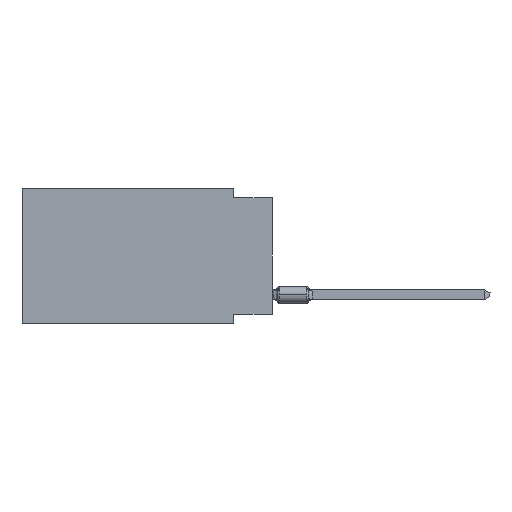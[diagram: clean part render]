
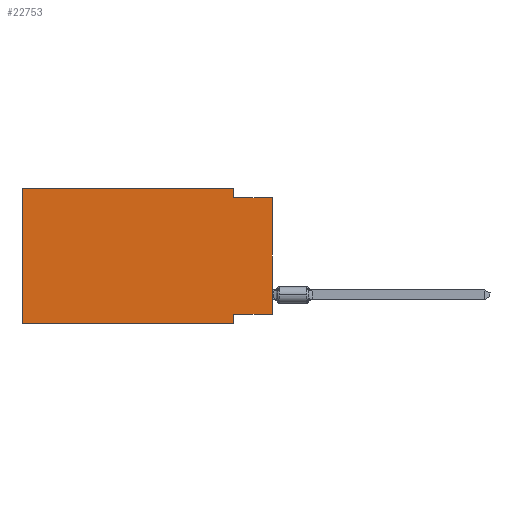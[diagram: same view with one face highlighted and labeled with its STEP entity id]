
A CAD part, left-side view. The second image highlights one B-rep face of the part: STEP entity #22753.
In plain terms, the highlighted planar face has unit normal (-1, 0, 0).
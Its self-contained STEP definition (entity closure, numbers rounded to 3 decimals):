
#332 = CARTESIAN_POINT ( 'NONE',  ( 0., 16.383, 0. ) ) ;
#1500 = ORIENTED_EDGE ( 'NONE', *, *, #2528, .T. ) ;
#1837 = VECTOR ( 'NONE', #15474, 1000. ) ;
#2460 = CARTESIAN_POINT ( 'NONE',  ( 0., 16.383, 0. ) ) ;
#2461 = VERTEX_POINT ( 'NONE', #23174 ) ;
#2528 = EDGE_CURVE ( 'NONE', #26982, #2461, #13024, .T. ) ;
#2749 = AXIS2_PLACEMENT_3D ( 'NONE', #332, #3429, #8899 ) ;
#3429 = DIRECTION ( 'NONE',  ( 1., 0., 0. ) ) ;
#3939 = DIRECTION ( 'NONE',  ( 0., -1., 0. ) ) ;
#4595 = DIRECTION ( 'NONE',  ( 0., 0., 1. ) ) ;
#4811 = VECTOR ( 'NONE', #4595, 1000. ) ;
#4900 = VERTEX_POINT ( 'NONE', #9694 ) ;
#5397 = CARTESIAN_POINT ( 'NONE',  ( 0., 0., -8.255 ) ) ;
#5995 = CARTESIAN_POINT ( 'NONE',  ( 0., 2.54, -8.89 ) ) ;
#6486 = EDGE_CURVE ( 'NONE', #4900, #34462, #22879, .T. ) ;
#7127 = ORIENTED_EDGE ( 'NONE', *, *, #11390, .F. ) ;
#7798 = VECTOR ( 'NONE', #11660, 1000. ) ;
#7998 = VECTOR ( 'NONE', #3939, 1000. ) ;
#8899 = DIRECTION ( 'NONE',  ( 0., 0., -1. ) ) ;
#9694 = CARTESIAN_POINT ( 'NONE',  ( 0., 2.54, -8.255 ) ) ;
#9794 = CARTESIAN_POINT ( 'NONE',  ( 0., 2.54, 0. ) ) ;
#10689 = VECTOR ( 'NONE', #33989, 1000. ) ;
#11288 = LINE ( 'NONE', #30801, #7798 ) ;
#11390 = EDGE_CURVE ( 'NONE', #14086, #2461, #34971, .T. ) ;
#11660 = DIRECTION ( 'NONE',  ( 0., 0., -1. ) ) ;
#11772 = LINE ( 'NONE', #5397, #16528 ) ;
#11944 = VERTEX_POINT ( 'NONE', #2460 ) ;
#12345 = EDGE_CURVE ( 'NONE', #11944, #24610, #33671, .T. ) ;
#12576 = EDGE_CURVE ( 'NONE', #30050, #34462, #32544, .T. ) ;
#13024 = LINE ( 'NONE', #13560, #20866 ) ;
#13560 = CARTESIAN_POINT ( 'NONE',  ( 0., 0., 0. ) ) ;
#14086 = VERTEX_POINT ( 'NONE', #18644 ) ;
#14142 = DIRECTION ( 'NONE',  ( 0., 1., 0. ) ) ;
#15474 = DIRECTION ( 'NONE',  ( 0., -1., 0. ) ) ;
#15601 = ORIENTED_EDGE ( 'NONE', *, *, #12345, .F. ) ;
#16215 = ORIENTED_EDGE ( 'NONE', *, *, #6486, .F. ) ;
#16327 = CARTESIAN_POINT ( 'NONE',  ( 0., 16.383, -8.89 ) ) ;
#16528 = VECTOR ( 'NONE', #14142, 1000. ) ;
#18141 = CARTESIAN_POINT ( 'NONE',  ( 0., 16.383, -8.89 ) ) ;
#18644 = CARTESIAN_POINT ( 'NONE',  ( 0., 2.54, -0.635 ) ) ;
#18817 = CARTESIAN_POINT ( 'NONE',  ( 0., 16.383, 0. ) ) ;
#18971 = EDGE_CURVE ( 'NONE', #26982, #4900, #11772, .T. ) ;
#19433 = ORIENTED_EDGE ( 'NONE', *, *, #27596, .F. ) ;
#19725 = ORIENTED_EDGE ( 'NONE', *, *, #12576, .T. ) ;
#20866 = VECTOR ( 'NONE', #30154, 1000. ) ;
#20907 = ORIENTED_EDGE ( 'NONE', *, *, #35634, .F. ) ;
#22368 = DIRECTION ( 'NONE',  ( 0., -1., 0. ) ) ;
#22753 = ADVANCED_FACE ( 'NONE', ( #34238 ), #31503, .F. ) ;
#22879 = LINE ( 'NONE', #28519, #10689 ) ;
#23174 = CARTESIAN_POINT ( 'NONE',  ( 0., 0., -0.635 ) ) ;
#24610 = VERTEX_POINT ( 'NONE', #9794 ) ;
#26982 = VERTEX_POINT ( 'NONE', #29265 ) ;
#27596 = EDGE_CURVE ( 'NONE', #30050, #11944, #32306, .T. ) ;
#27636 = CARTESIAN_POINT ( 'NONE',  ( 0., 16.383, 0. ) ) ;
#28519 = CARTESIAN_POINT ( 'NONE',  ( 0., 2.54, -8.89 ) ) ;
#29265 = CARTESIAN_POINT ( 'NONE',  ( 0., 0., -8.255 ) ) ;
#29875 = EDGE_LOOP ( 'NONE', ( #1500, #7127, #20907, #15601, #19433, #19725, #16215, #35993 ) ) ;
#30050 = VERTEX_POINT ( 'NONE', #16327 ) ;
#30154 = DIRECTION ( 'NONE',  ( 0., 0., 1. ) ) ;
#30801 = CARTESIAN_POINT ( 'NONE',  ( 0., 2.54, 0. ) ) ;
#31503 = PLANE ( 'NONE',  #2749 ) ;
#32306 = LINE ( 'NONE', #18817, #4811 ) ;
#32544 = LINE ( 'NONE', #18141, #7998 ) ;
#33671 = LINE ( 'NONE', #27636, #34160 ) ;
#33989 = DIRECTION ( 'NONE',  ( 0., 0., -1. ) ) ;
#34160 = VECTOR ( 'NONE', #22368, 1000. ) ;
#34238 = FACE_OUTER_BOUND ( 'NONE', #29875, .T. ) ;
#34261 = CARTESIAN_POINT ( 'NONE',  ( 0., 0., -0.635 ) ) ;
#34462 = VERTEX_POINT ( 'NONE', #5995 ) ;
#34971 = LINE ( 'NONE', #34261, #1837 ) ;
#35634 = EDGE_CURVE ( 'NONE', #24610, #14086, #11288, .T. ) ;
#35993 = ORIENTED_EDGE ( 'NONE', *, *, #18971, .F. ) ;
